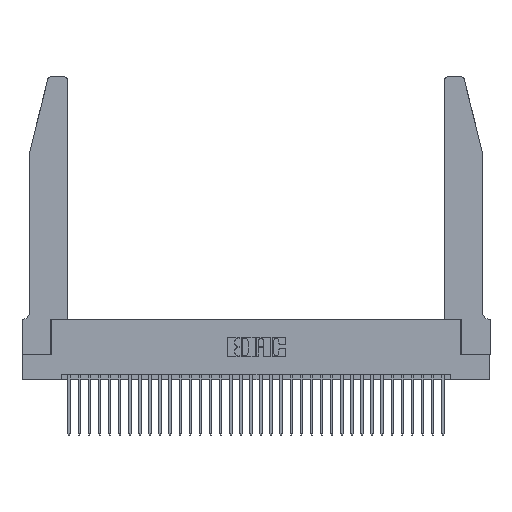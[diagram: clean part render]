
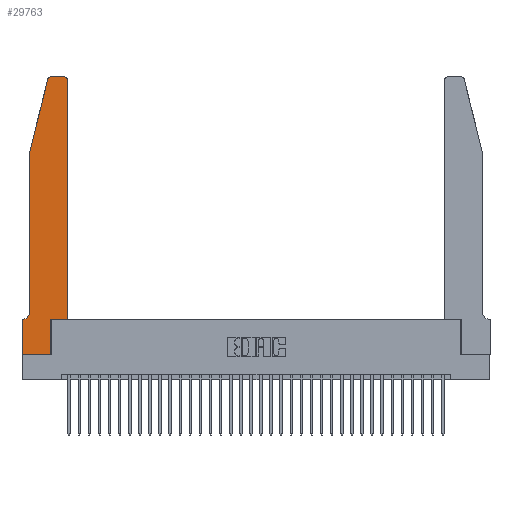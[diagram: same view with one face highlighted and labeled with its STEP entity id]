
A CAD part, top view. The second image highlights one B-rep face of the part: STEP entity #29763.
In plain terms, the highlighted planar face has unit normal (0, 0, 1).
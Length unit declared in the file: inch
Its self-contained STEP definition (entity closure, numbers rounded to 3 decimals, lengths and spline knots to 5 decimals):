
#648 = CARTESIAN_POINT ( 'NONE',  ( 0.0755, 0.42, 0.37 ) ) ;
#1343 = CARTESIAN_POINT ( 'NONE',  ( 0.4505, 0.35, 0.37 ) ) ;
#1424 = CARTESIAN_POINT ( 'NONE',  ( 0.2865, 0., 0.37 ) ) ;
#1481 = DIRECTION ( 'NONE',  ( 1., 0., 0. ) ) ;
#1977 = ORIENTED_EDGE ( 'NONE', *, *, #32276, .T. ) ;
#2464 = AXIS2_PLACEMENT_3D ( 'NONE', #14136, #32859, #16877 ) ;
#2647 = ORIENTED_EDGE ( 'NONE', *, *, #14012, .T. ) ;
#3116 = VECTOR ( 'NONE', #8279, 39.37008 ) ;
#3742 = VERTEX_POINT ( 'NONE', #22992 ) ;
#4188 = VERTEX_POINT ( 'NONE', #32465 ) ;
#4368 = VERTEX_POINT ( 'NONE', #648 ) ;
#4570 = EDGE_CURVE ( 'NONE', #4368, #10827, #15995, .T. ) ;
#4661 = VECTOR ( 'NONE', #25284, 39.37008 ) ;
#4917 = VECTOR ( 'NONE', #8156, 39.37008 ) ;
#4982 = EDGE_CURVE ( 'NONE', #16388, #3742, #9486, .T. ) ;
#5860 = CARTESIAN_POINT ( 'NONE',  ( 0.25487, 2.72718, 0.37 ) ) ;
#5911 = EDGE_CURVE ( 'NONE', #4188, #16388, #17590, .T. ) ;
#6248 = CARTESIAN_POINT ( 'NONE',  ( 0.2605, 2.75, 0.37 ) ) ;
#6261 = ORIENTED_EDGE ( 'NONE', *, *, #23685, .T. ) ;
#6655 = CARTESIAN_POINT ( 'NONE',  ( 0., 0., 0.37 ) ) ;
#6908 = CARTESIAN_POINT ( 'NONE',  ( 0., 0.35, 0.37 ) ) ;
#7069 = CARTESIAN_POINT ( 'NONE',  ( 0.0055, 0.42, 0.37 ) ) ;
#7403 = CARTESIAN_POINT ( 'NONE',  ( 0., 0., 0.37 ) ) ;
#8156 = DIRECTION ( 'NONE',  ( 0., 1., 0. ) ) ;
#8279 = DIRECTION ( 'NONE',  ( -0.239, -0.971, 0. ) ) ;
#9135 = AXIS2_PLACEMENT_3D ( 'NONE', #6908, #33927, #17973 ) ;
#9401 = EDGE_CURVE ( 'NONE', #16760, #4368, #25717, .T. ) ;
#9409 = VECTOR ( 'NONE', #31269, 39.37008 ) ;
#9486 = LINE ( 'NONE', #1343, #10364 ) ;
#9733 = ORIENTED_EDGE ( 'NONE', *, *, #14594, .T. ) ;
#9846 = DIRECTION ( 'NONE',  ( -1., 0., 0. ) ) ;
#10364 = VECTOR ( 'NONE', #20589, 39.37008 ) ;
#10472 = LINE ( 'NONE', #16479, #3116 ) ;
#10529 = LINE ( 'NONE', #32337, #4917 ) ;
#10827 = VERTEX_POINT ( 'NONE', #25558 ) ;
#11845 = EDGE_CURVE ( 'NONE', #30883, #16760, #10472, .T. ) ;
#12793 = ORIENTED_EDGE ( 'NONE', *, *, #15329, .T. ) ;
#13599 = VECTOR ( 'NONE', #23010, 39.37008 ) ;
#13742 = CIRCLE ( 'NONE', #23331, 0.03 ) ;
#14012 = EDGE_CURVE ( 'NONE', #3742, #19516, #13742, .T. ) ;
#14023 = CARTESIAN_POINT ( 'NONE',  ( 0.284, 2.75, 0.37 ) ) ;
#14136 = CARTESIAN_POINT ( 'NONE',  ( 0.284, 2.72, 0.37 ) ) ;
#14407 = VERTEX_POINT ( 'NONE', #27311 ) ;
#14594 = EDGE_CURVE ( 'NONE', #19516, #18707, #31730, .T. ) ;
#15144 = CARTESIAN_POINT ( 'NONE',  ( 0.0755, 0.35, 0.37 ) ) ;
#15222 = PLANE ( 'NONE',  #9135 ) ;
#15329 = EDGE_CURVE ( 'NONE', #10827, #14407, #25889, .T. ) ;
#15905 = EDGE_CURVE ( 'NONE', #14407, #21377, #35008, .T. ) ;
#15995 = CIRCLE ( 'NONE', #26487, 0.07 ) ;
#16388 = VERTEX_POINT ( 'NONE', #22857 ) ;
#16479 = CARTESIAN_POINT ( 'NONE',  ( 0.0755, 2., 0.37 ) ) ;
#16760 = VERTEX_POINT ( 'NONE', #27343 ) ;
#16877 = DIRECTION ( 'NONE',  ( 1., 0., 0. ) ) ;
#16982 = DIRECTION ( 'NONE',  ( 0., -1., 0. ) ) ;
#17590 = LINE ( 'NONE', #23283, #9409 ) ;
#17973 = DIRECTION ( 'NONE',  ( 1., 0., 0. ) ) ;
#18015 = DIRECTION ( 'NONE',  ( 0., 0., 1. ) ) ;
#18707 = VERTEX_POINT ( 'NONE', #14023 ) ;
#19288 = ORIENTED_EDGE ( 'NONE', *, *, #11845, .T. ) ;
#19516 = VERTEX_POINT ( 'NONE', #20646 ) ;
#20589 = DIRECTION ( 'NONE',  ( 0., 1., 0. ) ) ;
#20646 = CARTESIAN_POINT ( 'NONE',  ( 0.4205, 2.75, 0.37 ) ) ;
#20873 = VERTEX_POINT ( 'NONE', #1424 ) ;
#21377 = VERTEX_POINT ( 'NONE', #34353 ) ;
#22857 = CARTESIAN_POINT ( 'NONE',  ( 0.4505, 0.35, 0.37 ) ) ;
#22992 = CARTESIAN_POINT ( 'NONE',  ( 0.4505, 2.72, 0.37 ) ) ;
#23010 = DIRECTION ( 'NONE',  ( 0., -1., 0. ) ) ;
#23283 = CARTESIAN_POINT ( 'NONE',  ( 0.4505, 0.35, 0.37 ) ) ;
#23331 = AXIS2_PLACEMENT_3D ( 'NONE', #33974, #18015, #1481 ) ;
#23685 = EDGE_CURVE ( 'NONE', #20873, #4188, #10529, .T. ) ;
#23972 = ORIENTED_EDGE ( 'NONE', *, *, #9401, .T. ) ;
#24947 = CARTESIAN_POINT ( 'NONE',  ( 0.0755, 2., 0.37 ) ) ;
#25284 = DIRECTION ( 'NONE',  ( -1., 0., 0. ) ) ;
#25558 = CARTESIAN_POINT ( 'NONE',  ( 0.0055, 0.35, 0.37 ) ) ;
#25717 = LINE ( 'NONE', #24947, #31932 ) ;
#25889 = LINE ( 'NONE', #15144, #32097 ) ;
#26078 = DIRECTION ( 'NONE',  ( 0., 0., -1. ) ) ;
#26187 = ORIENTED_EDGE ( 'NONE', *, *, #15905, .T. ) ;
#26487 = AXIS2_PLACEMENT_3D ( 'NONE', #7069, #26078, #9846 ) ;
#26843 = ORIENTED_EDGE ( 'NONE', *, *, #4982, .T. ) ;
#27311 = CARTESIAN_POINT ( 'NONE',  ( 0., 0.35, 0.37 ) ) ;
#27343 = CARTESIAN_POINT ( 'NONE',  ( 0.0755, 2., 0.37 ) ) ;
#27621 = ORIENTED_EDGE ( 'NONE', *, *, #5911, .T. ) ;
#29763 = ADVANCED_FACE ( 'NONE', ( #32842 ), #15222, .T. ) ;
#30883 = VERTEX_POINT ( 'NONE', #5860 ) ;
#31009 = VECTOR ( 'NONE', #34414, 39.37008 ) ;
#31047 = DIRECTION ( 'NONE',  ( -1., 0., 0. ) ) ;
#31269 = DIRECTION ( 'NONE',  ( 1., 0., 0. ) ) ;
#31730 = LINE ( 'NONE', #6248, #4661 ) ;
#31844 = LINE ( 'NONE', #7403, #31009 ) ;
#31932 = VECTOR ( 'NONE', #16982, 39.37008 ) ;
#32066 = EDGE_CURVE ( 'NONE', #21377, #20873, #31844, .T. ) ;
#32097 = VECTOR ( 'NONE', #31047, 39.37008 ) ;
#32276 = EDGE_CURVE ( 'NONE', #18707, #30883, #33079, .T. ) ;
#32337 = CARTESIAN_POINT ( 'NONE',  ( 0.2865, 0.35, 0.37 ) ) ;
#32465 = CARTESIAN_POINT ( 'NONE',  ( 0.2865, 0.35, 0.37 ) ) ;
#32832 = ORIENTED_EDGE ( 'NONE', *, *, #32066, .T. ) ;
#32842 = FACE_OUTER_BOUND ( 'NONE', #34571, .T. ) ;
#32859 = DIRECTION ( 'NONE',  ( 0., 0., 1. ) ) ;
#32891 = ORIENTED_EDGE ( 'NONE', *, *, #4570, .T. ) ;
#33079 = CIRCLE ( 'NONE', #2464, 0.03 ) ;
#33927 = DIRECTION ( 'NONE',  ( 0., 0., 1. ) ) ;
#33974 = CARTESIAN_POINT ( 'NONE',  ( 0.4205, 2.72, 0.37 ) ) ;
#34353 = CARTESIAN_POINT ( 'NONE',  ( 0., 0., 0.37 ) ) ;
#34414 = DIRECTION ( 'NONE',  ( 1., 0., 0. ) ) ;
#34571 = EDGE_LOOP ( 'NONE', ( #9733, #1977, #19288, #23972, #32891, #12793, #26187, #32832, #6261, #27621, #26843, #2647 ) ) ;
#35008 = LINE ( 'NONE', #6655, #13599 ) ;
